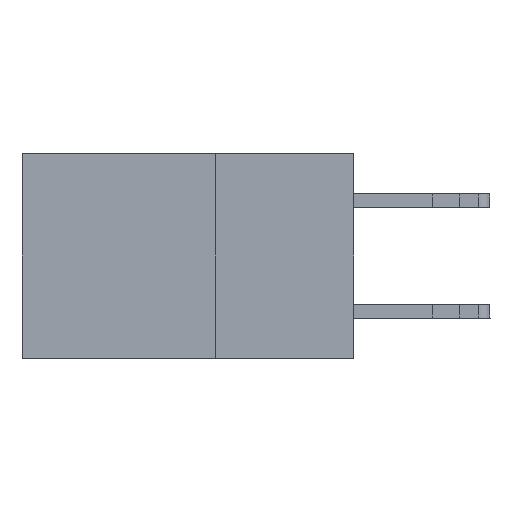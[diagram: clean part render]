
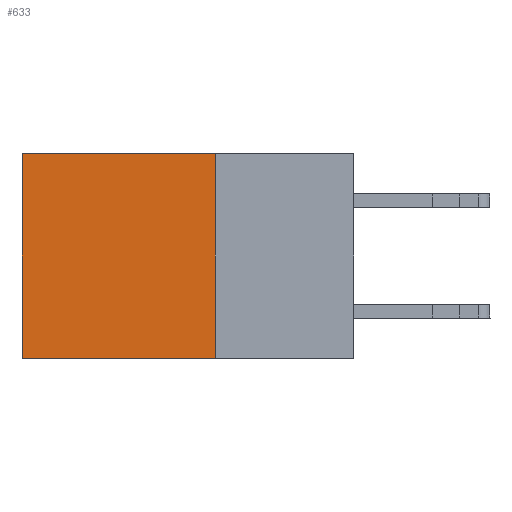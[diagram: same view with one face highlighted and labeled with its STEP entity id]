
A CAD part, left-side view. The second image highlights one B-rep face of the part: STEP entity #633.
In plain terms, the highlighted planar face has unit normal (-1, 0, 0).
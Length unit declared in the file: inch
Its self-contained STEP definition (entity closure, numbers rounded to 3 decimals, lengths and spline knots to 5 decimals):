
#529 = ORIENTED_EDGE ( 'NONE', *, *, #2927, .T. ) ;
#633 = ADVANCED_FACE ( 'NONE', ( #7025 ), #7251, .F. ) ;
#1556 = CARTESIAN_POINT ( 'NONE',  ( 0.2875, 0.25, -0.37 ) ) ;
#1856 = DIRECTION ( 'NONE',  ( 0., 0., -1. ) ) ;
#2927 = EDGE_CURVE ( 'NONE', #9737, #16594, #18677, .T. ) ;
#3031 = LINE ( 'NONE', #14985, #8614 ) ;
#3088 = VERTEX_POINT ( 'NONE', #1556 ) ;
#3564 = AXIS2_PLACEMENT_3D ( 'NONE', #6912, #3744, #1856 ) ;
#3681 = CARTESIAN_POINT ( 'NONE',  ( 0.2875, 0.6, -0.37 ) ) ;
#3744 = DIRECTION ( 'NONE',  ( 1., 0., 0. ) ) ;
#5164 = ORIENTED_EDGE ( 'NONE', *, *, #5678, .F. ) ;
#5569 = CARTESIAN_POINT ( 'NONE',  ( 0.2875, 0.6, 0. ) ) ;
#5678 = EDGE_CURVE ( 'NONE', #3088, #16594, #3031, .T. ) ;
#6453 = EDGE_CURVE ( 'NONE', #13444, #3088, #14125, .T. ) ;
#6488 = DIRECTION ( 'NONE',  ( 0., 0., -1. ) ) ;
#6912 = CARTESIAN_POINT ( 'NONE',  ( 0.2875, 0.25, 0. ) ) ;
#7025 = FACE_OUTER_BOUND ( 'NONE', #12431, .T. ) ;
#7251 = PLANE ( 'NONE',  #3564 ) ;
#7797 = EDGE_CURVE ( 'NONE', #13444, #9737, #15539, .T. ) ;
#8008 = DIRECTION ( 'NONE',  ( 0., 1., 0. ) ) ;
#8317 = CARTESIAN_POINT ( 'NONE',  ( 0.2875, 0.6, 0. ) ) ;
#8390 = VECTOR ( 'NONE', #6488, 39.37008 ) ;
#8614 = VECTOR ( 'NONE', #8008, 39.37008 ) ;
#8974 = DIRECTION ( 'NONE',  ( 0., 0., -1. ) ) ;
#9737 = VERTEX_POINT ( 'NONE', #5569 ) ;
#10044 = CARTESIAN_POINT ( 'NONE',  ( 0.2875, 0.25, 0. ) ) ;
#11438 = VECTOR ( 'NONE', #8974, 39.37008 ) ;
#11545 = ORIENTED_EDGE ( 'NONE', *, *, #6453, .F. ) ;
#12162 = CARTESIAN_POINT ( 'NONE',  ( 0.2875, 0.25, 0. ) ) ;
#12431 = EDGE_LOOP ( 'NONE', ( #529, #5164, #11545, #19739 ) ) ;
#12578 = VECTOR ( 'NONE', #15308, 39.37008 ) ;
#12947 = CARTESIAN_POINT ( 'NONE',  ( 0.2875, 0.25, 0. ) ) ;
#13444 = VERTEX_POINT ( 'NONE', #12947 ) ;
#14125 = LINE ( 'NONE', #12162, #11438 ) ;
#14985 = CARTESIAN_POINT ( 'NONE',  ( 0.2875, 0.25, -0.37 ) ) ;
#15308 = DIRECTION ( 'NONE',  ( 0., 1., 0. ) ) ;
#15539 = LINE ( 'NONE', #10044, #12578 ) ;
#16594 = VERTEX_POINT ( 'NONE', #3681 ) ;
#18677 = LINE ( 'NONE', #8317, #8390 ) ;
#19739 = ORIENTED_EDGE ( 'NONE', *, *, #7797, .T. ) ;
